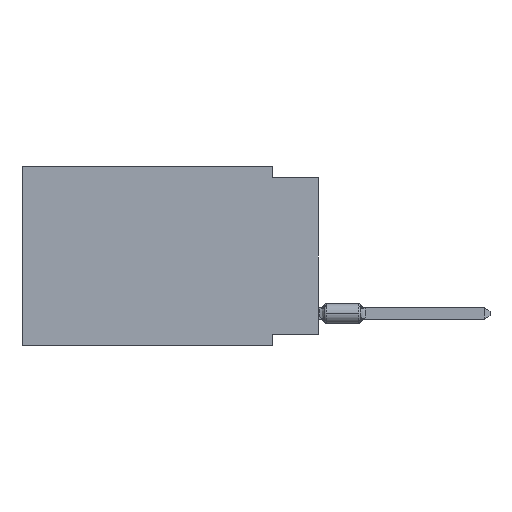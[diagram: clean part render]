
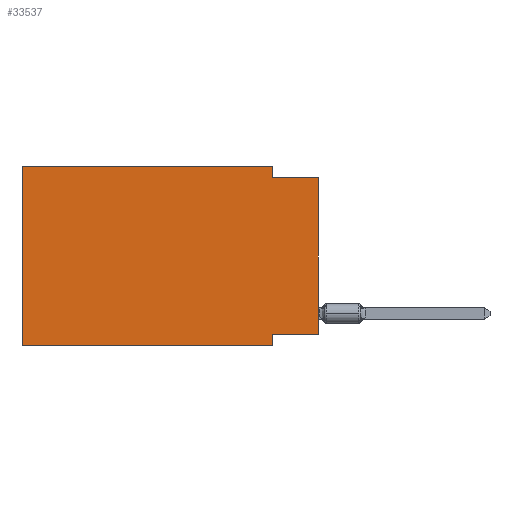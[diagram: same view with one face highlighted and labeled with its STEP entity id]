
A CAD part, left-side view. The second image highlights one B-rep face of the part: STEP entity #33537.
In plain terms, the highlighted planar face has unit normal (-1, 0, 0).
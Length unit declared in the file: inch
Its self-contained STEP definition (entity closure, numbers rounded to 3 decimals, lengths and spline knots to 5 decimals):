
#678 = LINE ( 'NONE', #15173, #7305 ) ;
#961 = VECTOR ( 'NONE', #45401, 39.37008 ) ;
#1096 = CARTESIAN_POINT ( 'NONE',  ( 0., 0.645, 0. ) ) ;
#1864 = CARTESIAN_POINT ( 'NONE',  ( 0., 0.1, -0.025 ) ) ;
#3028 = DIRECTION ( 'NONE',  ( 0., 0., -1. ) ) ;
#3044 = VECTOR ( 'NONE', #23136, 39.37008 ) ;
#4102 = VERTEX_POINT ( 'NONE', #44446 ) ;
#4110 = CARTESIAN_POINT ( 'NONE',  ( 0., 0., -0.365 ) ) ;
#5087 = DIRECTION ( 'NONE',  ( 1., 0., 0. ) ) ;
#5920 = ORIENTED_EDGE ( 'NONE', *, *, #6576, .T. ) ;
#6365 = CARTESIAN_POINT ( 'NONE',  ( 0., 0.1, 0. ) ) ;
#6576 = EDGE_CURVE ( 'NONE', #8023, #18628, #34097, .T. ) ;
#7305 = VECTOR ( 'NONE', #27526, 39.37008 ) ;
#8023 = VERTEX_POINT ( 'NONE', #4110 ) ;
#8876 = FACE_OUTER_BOUND ( 'NONE', #37301, .T. ) ;
#9187 = VECTOR ( 'NONE', #28305, 39.37008 ) ;
#10129 = EDGE_CURVE ( 'NONE', #8023, #20777, #29934, .T. ) ;
#11209 = ORIENTED_EDGE ( 'NONE', *, *, #22893, .T. ) ;
#12319 = VERTEX_POINT ( 'NONE', #32883 ) ;
#12344 = CARTESIAN_POINT ( 'NONE',  ( 0., 0., -0.365 ) ) ;
#13277 = ORIENTED_EDGE ( 'NONE', *, *, #10129, .F. ) ;
#13278 = LINE ( 'NONE', #6365, #18797 ) ;
#13283 = ORIENTED_EDGE ( 'NONE', *, *, #26827, .F. ) ;
#15173 = CARTESIAN_POINT ( 'NONE',  ( 0., 0.1, -0.39 ) ) ;
#16876 = CARTESIAN_POINT ( 'NONE',  ( 0., 0., -0.025 ) ) ;
#16902 = ORIENTED_EDGE ( 'NONE', *, *, #19219, .F. ) ;
#18628 = VERTEX_POINT ( 'NONE', #16876 ) ;
#18797 = VECTOR ( 'NONE', #3028, 39.37008 ) ;
#19219 = EDGE_CURVE ( 'NONE', #22036, #30848, #13278, .T. ) ;
#20441 = LINE ( 'NONE', #27607, #9187 ) ;
#20777 = VERTEX_POINT ( 'NONE', #45580 ) ;
#22036 = VERTEX_POINT ( 'NONE', #30907 ) ;
#22663 = DIRECTION ( 'NONE',  ( 0., -1., 0. ) ) ;
#22893 = EDGE_CURVE ( 'NONE', #33450, #4102, #44787, .T. ) ;
#23136 = DIRECTION ( 'NONE',  ( 0., -1., 0. ) ) ;
#23370 = CARTESIAN_POINT ( 'NONE',  ( 0., 0.645, 0. ) ) ;
#26827 = EDGE_CURVE ( 'NONE', #33450, #12319, #29623, .T. ) ;
#27033 = VECTOR ( 'NONE', #22663, 39.37008 ) ;
#27526 = DIRECTION ( 'NONE',  ( 0., 0., -1. ) ) ;
#27607 = CARTESIAN_POINT ( 'NONE',  ( 0., 0.645, 0. ) ) ;
#28305 = DIRECTION ( 'NONE',  ( 0., -1., 0. ) ) ;
#29340 = ORIENTED_EDGE ( 'NONE', *, *, #44760, .F. ) ;
#29623 = LINE ( 'NONE', #1096, #45015 ) ;
#29859 = ORIENTED_EDGE ( 'NONE', *, *, #32723, .F. ) ;
#29934 = LINE ( 'NONE', #12344, #961 ) ;
#30848 = VERTEX_POINT ( 'NONE', #1864 ) ;
#30907 = CARTESIAN_POINT ( 'NONE',  ( 0., 0.1, 0. ) ) ;
#32723 = EDGE_CURVE ( 'NONE', #30848, #18628, #33608, .T. ) ;
#32883 = CARTESIAN_POINT ( 'NONE',  ( 0., 0.645, 0. ) ) ;
#33450 = VERTEX_POINT ( 'NONE', #40994 ) ;
#33537 = ADVANCED_FACE ( 'NONE', ( #8876 ), #41234, .F. ) ;
#33608 = LINE ( 'NONE', #34323, #27033 ) ;
#34097 = LINE ( 'NONE', #44805, #38055 ) ;
#34318 = CARTESIAN_POINT ( 'NONE',  ( 0., 0.645, -0.39 ) ) ;
#34319 = DIRECTION ( 'NONE',  ( 0., 0., -1. ) ) ;
#34323 = CARTESIAN_POINT ( 'NONE',  ( 0., 0., -0.025 ) ) ;
#34805 = DIRECTION ( 'NONE',  ( 0., 0., 1. ) ) ;
#36545 = EDGE_CURVE ( 'NONE', #12319, #22036, #20441, .T. ) ;
#37301 = EDGE_LOOP ( 'NONE', ( #5920, #29859, #16902, #41502, #13283, #11209, #29340, #13277 ) ) ;
#38055 = VECTOR ( 'NONE', #34805, 39.37008 ) ;
#39994 = AXIS2_PLACEMENT_3D ( 'NONE', #23370, #5087, #34319 ) ;
#40994 = CARTESIAN_POINT ( 'NONE',  ( 0., 0.645, -0.39 ) ) ;
#41234 = PLANE ( 'NONE',  #39994 ) ;
#41290 = DIRECTION ( 'NONE',  ( 0., 0., 1. ) ) ;
#41502 = ORIENTED_EDGE ( 'NONE', *, *, #36545, .F. ) ;
#44446 = CARTESIAN_POINT ( 'NONE',  ( 0., 0.1, -0.39 ) ) ;
#44760 = EDGE_CURVE ( 'NONE', #20777, #4102, #678, .T. ) ;
#44787 = LINE ( 'NONE', #34318, #3044 ) ;
#44805 = CARTESIAN_POINT ( 'NONE',  ( 0., 0., 0. ) ) ;
#45015 = VECTOR ( 'NONE', #41290, 39.37008 ) ;
#45401 = DIRECTION ( 'NONE',  ( 0., 1., 0. ) ) ;
#45580 = CARTESIAN_POINT ( 'NONE',  ( 0., 0.1, -0.365 ) ) ;
